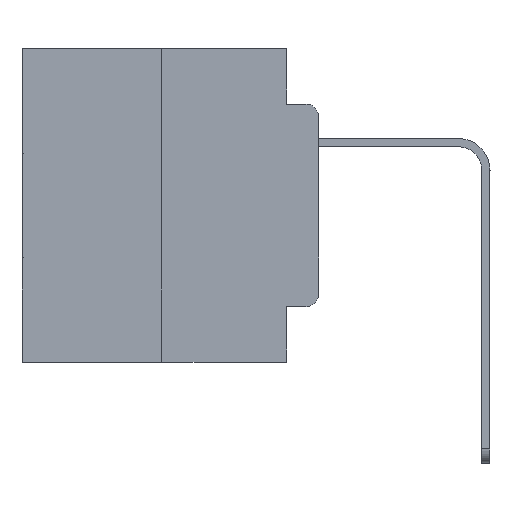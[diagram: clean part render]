
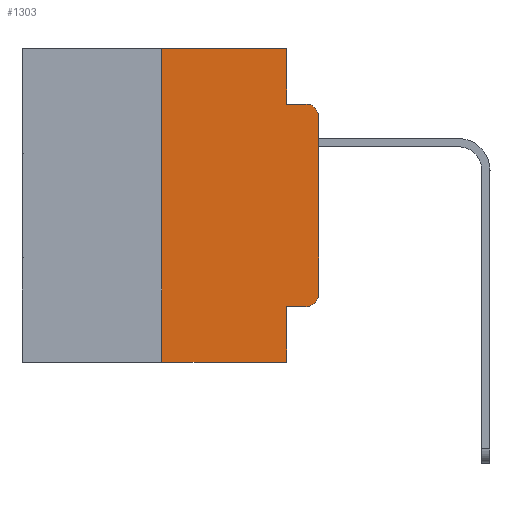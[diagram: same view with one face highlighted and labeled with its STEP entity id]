
A CAD part, left-side view. The second image highlights one B-rep face of the part: STEP entity #1303.
In plain terms, the highlighted planar face has unit normal (-1, 0, 0).
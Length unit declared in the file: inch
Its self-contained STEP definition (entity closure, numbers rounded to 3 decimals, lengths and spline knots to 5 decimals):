
#373 = VERTEX_POINT ( 'NONE', #20118 ) ;
#1060 = LINE ( 'NONE', #18489, #2979 ) ;
#1303 = ADVANCED_FACE ( 'NONE', ( #11438 ), #22933, .F. ) ;
#1721 = ORIENTED_EDGE ( 'NONE', *, *, #22494, .T. ) ;
#1838 = EDGE_CURVE ( 'NONE', #20553, #20030, #7848, .T. ) ;
#2143 = VERTEX_POINT ( 'NONE', #11482 ) ;
#2169 = DIRECTION ( 'NONE',  ( 0., -1., 0. ) ) ;
#2506 = ORIENTED_EDGE ( 'NONE', *, *, #16493, .T. ) ;
#2735 = CARTESIAN_POINT ( 'NONE',  ( 0., 0.051, -0.4115 ) ) ;
#2953 = EDGE_CURVE ( 'NONE', #15849, #16643, #6485, .T. ) ;
#2979 = VECTOR ( 'NONE', #14164, 39.37008 ) ;
#3150 = VECTOR ( 'NONE', #5383, 39.37008 ) ;
#3262 = LINE ( 'NONE', #17483, #18988 ) ;
#3550 = DIRECTION ( 'NONE',  ( 0., -1., 0. ) ) ;
#3576 = ORIENTED_EDGE ( 'NONE', *, *, #24853, .T. ) ;
#3746 = CARTESIAN_POINT ( 'NONE',  ( 0., 0.02, -0.3915 ) ) ;
#3752 = ORIENTED_EDGE ( 'NONE', *, *, #22688, .F. ) ;
#3972 = AXIS2_PLACEMENT_3D ( 'NONE', #18816, #24908, #12875 ) ;
#5383 = DIRECTION ( 'NONE',  ( 0., 0., 1. ) ) ;
#5478 = VERTEX_POINT ( 'NONE', #2735 ) ;
#5913 = DIRECTION ( 'NONE',  ( 0., -1., 0. ) ) ;
#6050 = CARTESIAN_POINT ( 'NONE',  ( 0., 0.25, 0. ) ) ;
#6485 = CIRCLE ( 'NONE', #10325, 0.02 ) ;
#7291 = EDGE_LOOP ( 'NONE', ( #3576, #2506, #15855, #18223, #3752, #14785, #1721, #18502, #13288, #8239 ) ) ;
#7848 = LINE ( 'NONE', #6050, #21998 ) ;
#8239 = ORIENTED_EDGE ( 'NONE', *, *, #2953, .T. ) ;
#8296 = VERTEX_POINT ( 'NONE', #14003 ) ;
#8356 = CIRCLE ( 'NONE', #26361, 0.02 ) ;
#9140 = VECTOR ( 'NONE', #3550, 39.37008 ) ;
#9690 = LINE ( 'NONE', #20738, #16095 ) ;
#10325 = AXIS2_PLACEMENT_3D ( 'NONE', #3746, #14050, #24464 ) ;
#10430 = CARTESIAN_POINT ( 'NONE',  ( 0., 0.25, 0. ) ) ;
#10455 = VERTEX_POINT ( 'NONE', #23350 ) ;
#11438 = FACE_OUTER_BOUND ( 'NONE', #7291, .T. ) ;
#11451 = CARTESIAN_POINT ( 'NONE',  ( 0., 0., 0. ) ) ;
#11482 = CARTESIAN_POINT ( 'NONE',  ( 0., 0.051, 0. ) ) ;
#11713 = LINE ( 'NONE', #21770, #9140 ) ;
#11799 = DIRECTION ( 'NONE',  ( 0., 0., -1. ) ) ;
#12875 = DIRECTION ( 'NONE',  ( 0., 0., -1. ) ) ;
#13023 = DIRECTION ( 'NONE',  ( 0., 0., -1. ) ) ;
#13288 = ORIENTED_EDGE ( 'NONE', *, *, #22957, .T. ) ;
#13419 = LINE ( 'NONE', #11451, #3150 ) ;
#14003 = CARTESIAN_POINT ( 'NONE',  ( 0., 0.051, -0.5 ) ) ;
#14050 = DIRECTION ( 'NONE',  ( -1., 0., 0. ) ) ;
#14164 = DIRECTION ( 'NONE',  ( 0., -1., 0. ) ) ;
#14785 = ORIENTED_EDGE ( 'NONE', *, *, #1838, .F. ) ;
#15354 = EDGE_CURVE ( 'NONE', #5478, #8296, #16439, .T. ) ;
#15849 = VERTEX_POINT ( 'NONE', #19707 ) ;
#15855 = ORIENTED_EDGE ( 'NONE', *, *, #16707, .F. ) ;
#16095 = VECTOR ( 'NONE', #2169, 39.37008 ) ;
#16103 = CARTESIAN_POINT ( 'NONE',  ( 0., 0.051, 0. ) ) ;
#16140 = CARTESIAN_POINT ( 'NONE',  ( 0., 0.25, -0.5 ) ) ;
#16439 = LINE ( 'NONE', #16103, #17072 ) ;
#16493 = EDGE_CURVE ( 'NONE', #10455, #373, #8356, .T. ) ;
#16643 = VERTEX_POINT ( 'NONE', #26163 ) ;
#16707 = EDGE_CURVE ( 'NONE', #24577, #373, #11713, .T. ) ;
#17072 = VECTOR ( 'NONE', #11799, 39.37008 ) ;
#17483 = CARTESIAN_POINT ( 'NONE',  ( 0., 0.051, -0.4115 ) ) ;
#18223 = ORIENTED_EDGE ( 'NONE', *, *, #25940, .F. ) ;
#18489 = CARTESIAN_POINT ( 'NONE',  ( 0., 0.473, -0.5 ) ) ;
#18502 = ORIENTED_EDGE ( 'NONE', *, *, #15354, .F. ) ;
#18816 = CARTESIAN_POINT ( 'NONE',  ( 0., 0.473, 0. ) ) ;
#18988 = VECTOR ( 'NONE', #5913, 39.37008 ) ;
#19707 = CARTESIAN_POINT ( 'NONE',  ( 0., 0.02, -0.4115 ) ) ;
#20030 = VERTEX_POINT ( 'NONE', #10430 ) ;
#20118 = CARTESIAN_POINT ( 'NONE',  ( 0., 0.02, -0.0885 ) ) ;
#20553 = VERTEX_POINT ( 'NONE', #16140 ) ;
#20738 = CARTESIAN_POINT ( 'NONE',  ( 0., 0.473, 0. ) ) ;
#21500 = DIRECTION ( 'NONE',  ( 0., 0., -1. ) ) ;
#21770 = CARTESIAN_POINT ( 'NONE',  ( 0., 0.051, -0.0885 ) ) ;
#21998 = VECTOR ( 'NONE', #22193, 39.37008 ) ;
#22193 = DIRECTION ( 'NONE',  ( 0., 0., 1. ) ) ;
#22494 = EDGE_CURVE ( 'NONE', #20553, #8296, #1060, .T. ) ;
#22688 = EDGE_CURVE ( 'NONE', #20030, #2143, #9690, .T. ) ;
#22933 = PLANE ( 'NONE',  #3972 ) ;
#22957 = EDGE_CURVE ( 'NONE', #5478, #15849, #3262, .T. ) ;
#23303 = LINE ( 'NONE', #25576, #23953 ) ;
#23350 = CARTESIAN_POINT ( 'NONE',  ( 0., 0., -0.1085 ) ) ;
#23387 = DIRECTION ( 'NONE',  ( -1., 0., 0. ) ) ;
#23750 = CARTESIAN_POINT ( 'NONE',  ( 0., 0.02, -0.1085 ) ) ;
#23953 = VECTOR ( 'NONE', #13023, 39.37008 ) ;
#24306 = CARTESIAN_POINT ( 'NONE',  ( 0., 0.051, -0.0885 ) ) ;
#24464 = DIRECTION ( 'NONE',  ( 0., 0., -1. ) ) ;
#24577 = VERTEX_POINT ( 'NONE', #24306 ) ;
#24853 = EDGE_CURVE ( 'NONE', #16643, #10455, #13419, .T. ) ;
#24908 = DIRECTION ( 'NONE',  ( 1., 0., 0. ) ) ;
#25576 = CARTESIAN_POINT ( 'NONE',  ( 0., 0.051, 0. ) ) ;
#25940 = EDGE_CURVE ( 'NONE', #2143, #24577, #23303, .T. ) ;
#26163 = CARTESIAN_POINT ( 'NONE',  ( 0., 0., -0.3915 ) ) ;
#26361 = AXIS2_PLACEMENT_3D ( 'NONE', #23750, #23387, #21500 ) ;
